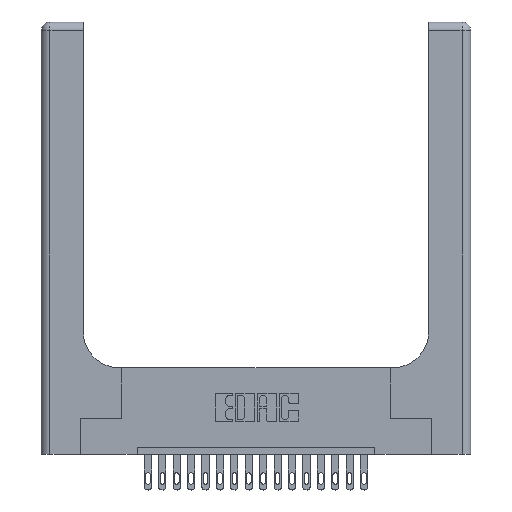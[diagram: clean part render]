
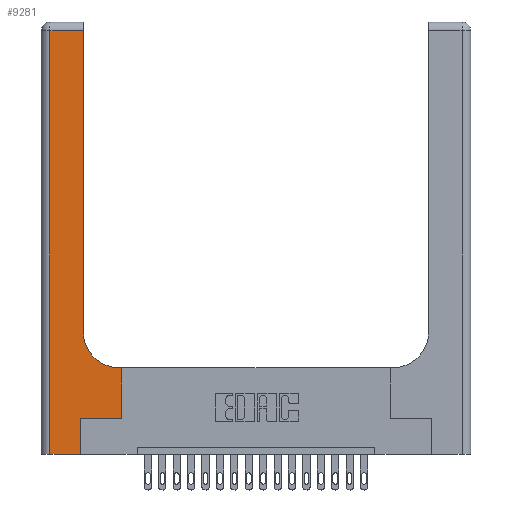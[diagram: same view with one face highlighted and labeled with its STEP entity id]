
A CAD part, top view. The second image highlights one B-rep face of the part: STEP entity #9281.
In plain terms, the highlighted planar face has unit normal (0, 0, 1).
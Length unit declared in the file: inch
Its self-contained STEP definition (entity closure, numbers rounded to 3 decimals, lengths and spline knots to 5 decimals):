
#322 = PLANE ( 'NONE',  #10365 ) ;
#713 = VERTEX_POINT ( 'NONE', #15528 ) ;
#758 = VERTEX_POINT ( 'NONE', #18724 ) ;
#878 = DIRECTION ( 'NONE',  ( 0., 1., 0. ) ) ;
#1083 = CARTESIAN_POINT ( 'NONE',  ( 0.5415, 0.85, 0.37 ) ) ;
#1428 = ORIENTED_EDGE ( 'NONE', *, *, #3490, .T. ) ;
#1854 = DIRECTION ( 'NONE',  ( -1., 0., 0. ) ) ;
#2239 = EDGE_LOOP ( 'NONE', ( #4079, #18112, #10687, #13114, #1428, #9887, #20367, #6157, #14821 ) ) ;
#2542 = LINE ( 'NONE', #8230, #19274 ) ;
#3162 = LINE ( 'NONE', #14872, #19125 ) ;
#3179 = EDGE_CURVE ( 'NONE', #18244, #19946, #20269, .T. ) ;
#3490 = EDGE_CURVE ( 'NONE', #713, #18244, #19019, .T. ) ;
#3637 = VERTEX_POINT ( 'NONE', #15131 ) ;
#3753 = EDGE_CURVE ( 'NONE', #11318, #758, #2542, .T. ) ;
#3851 = FACE_OUTER_BOUND ( 'NONE', #2239, .T. ) ;
#4079 = ORIENTED_EDGE ( 'NONE', *, *, #3753, .T. ) ;
#4220 = LINE ( 'NONE', #6350, #6248 ) ;
#4370 = DIRECTION ( 'NONE',  ( 0., 0., -1. ) ) ;
#4493 = LINE ( 'NONE', #16743, #4980 ) ;
#4513 = DIRECTION ( 'NONE',  ( 1., 0., 0. ) ) ;
#4980 = VECTOR ( 'NONE', #7200, 39.37008 ) ;
#5228 = CARTESIAN_POINT ( 'NONE',  ( 0.06, 0., 0.37 ) ) ;
#5419 = EDGE_CURVE ( 'NONE', #19946, #3637, #4493, .T. ) ;
#5727 = EDGE_CURVE ( 'NONE', #758, #8691, #18176, .T. ) ;
#5981 = VECTOR ( 'NONE', #4513, 39.37008 ) ;
#6157 = ORIENTED_EDGE ( 'NONE', *, *, #16268, .T. ) ;
#6222 = EDGE_CURVE ( 'NONE', #15549, #11318, #14431, .T. ) ;
#6248 = VECTOR ( 'NONE', #14364, 39.37008 ) ;
#6350 = CARTESIAN_POINT ( 'NONE',  ( 0.06, 3., 0.37 ) ) ;
#6728 = CARTESIAN_POINT ( 'NONE',  ( 0.5585, 0.25, 0.37 ) ) ;
#7200 = DIRECTION ( 'NONE',  ( 0., 1., 0. ) ) ;
#8230 = CARTESIAN_POINT ( 'NONE',  ( 0.2915, 3., 0.37 ) ) ;
#8564 = CARTESIAN_POINT ( 'NONE',  ( 0.2915, 0.85, 0.37 ) ) ;
#8691 = VERTEX_POINT ( 'NONE', #16197 ) ;
#8937 = DIRECTION ( 'NONE',  ( -1., 0., 0. ) ) ;
#9048 = VECTOR ( 'NONE', #16724, 39.37008 ) ;
#9281 = ADVANCED_FACE ( 'NONE', ( #3851 ), #322, .F. ) ;
#9696 = DIRECTION ( 'NONE',  ( -1., 0., 0. ) ) ;
#9887 = ORIENTED_EDGE ( 'NONE', *, *, #3179, .T. ) ;
#10149 = DIRECTION ( 'NONE',  ( 0., 1., 0. ) ) ;
#10365 = AXIS2_PLACEMENT_3D ( 'NONE', #11619, #19423, #1854 ) ;
#10687 = ORIENTED_EDGE ( 'NONE', *, *, #12464, .T. ) ;
#10703 = DIRECTION ( 'NONE',  ( 1., 0., 0. ) ) ;
#10927 = CARTESIAN_POINT ( 'NONE',  ( 0.5415, 0.6, 0.37 ) ) ;
#11318 = VERTEX_POINT ( 'NONE', #8564 ) ;
#11619 = CARTESIAN_POINT ( 'NONE',  ( 0., 3., 0.37 ) ) ;
#12241 = CARTESIAN_POINT ( 'NONE',  ( 0., 0., 0.37 ) ) ;
#12464 = EDGE_CURVE ( 'NONE', #8691, #18718, #4220, .T. ) ;
#12469 = LINE ( 'NONE', #12241, #5981 ) ;
#12762 = EDGE_CURVE ( 'NONE', #18718, #713, #12469, .T. ) ;
#13114 = ORIENTED_EDGE ( 'NONE', *, *, #12762, .T. ) ;
#13958 = VECTOR ( 'NONE', #8937, 39.37008 ) ;
#14364 = DIRECTION ( 'NONE',  ( 0., -1., 0. ) ) ;
#14431 = CIRCLE ( 'NONE', #16118, 0.25 ) ;
#14821 = ORIENTED_EDGE ( 'NONE', *, *, #6222, .T. ) ;
#14872 = CARTESIAN_POINT ( 'NONE',  ( 0.2915, 0.6, 0.37 ) ) ;
#15131 = CARTESIAN_POINT ( 'NONE',  ( 0.5585, 0.6, 0.37 ) ) ;
#15528 = CARTESIAN_POINT ( 'NONE',  ( 0.269, 0., 0.37 ) ) ;
#15549 = VERTEX_POINT ( 'NONE', #10927 ) ;
#16118 = AXIS2_PLACEMENT_3D ( 'NONE', #1083, #4370, #10703 ) ;
#16197 = CARTESIAN_POINT ( 'NONE',  ( 0.06, 2.94, 0.37 ) ) ;
#16267 = VECTOR ( 'NONE', #10149, 39.37008 ) ;
#16268 = EDGE_CURVE ( 'NONE', #3637, #15549, #3162, .T. ) ;
#16524 = CARTESIAN_POINT ( 'NONE',  ( 0.269, 0., 0.37 ) ) ;
#16724 = DIRECTION ( 'NONE',  ( 1., 0., 0. ) ) ;
#16743 = CARTESIAN_POINT ( 'NONE',  ( 0.5585, 0.25, 0.37 ) ) ;
#18112 = ORIENTED_EDGE ( 'NONE', *, *, #5727, .T. ) ;
#18176 = LINE ( 'NONE', #18765, #13958 ) ;
#18244 = VERTEX_POINT ( 'NONE', #20013 ) ;
#18718 = VERTEX_POINT ( 'NONE', #5228 ) ;
#18724 = CARTESIAN_POINT ( 'NONE',  ( 0.2915, 2.94, 0.37 ) ) ;
#18765 = CARTESIAN_POINT ( 'NONE',  ( 0., 2.94, 0.37 ) ) ;
#19019 = LINE ( 'NONE', #16524, #16267 ) ;
#19125 = VECTOR ( 'NONE', #9696, 39.37008 ) ;
#19274 = VECTOR ( 'NONE', #878, 39.37008 ) ;
#19423 = DIRECTION ( 'NONE',  ( 0., 0., -1. ) ) ;
#19852 = CARTESIAN_POINT ( 'NONE',  ( 0.269, 0.25, 0.37 ) ) ;
#19946 = VERTEX_POINT ( 'NONE', #6728 ) ;
#20013 = CARTESIAN_POINT ( 'NONE',  ( 0.269, 0.25, 0.37 ) ) ;
#20269 = LINE ( 'NONE', #19852, #9048 ) ;
#20367 = ORIENTED_EDGE ( 'NONE', *, *, #5419, .T. ) ;
